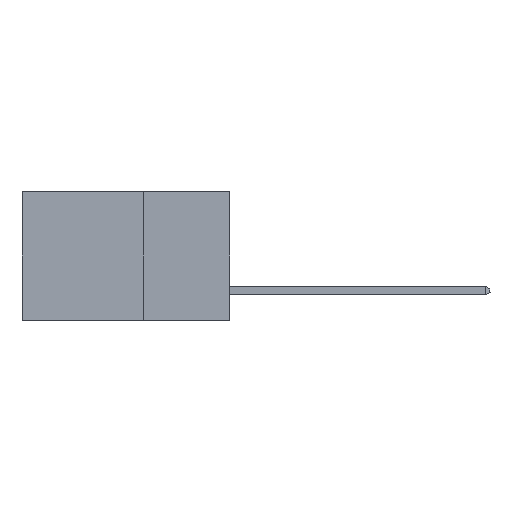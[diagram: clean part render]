
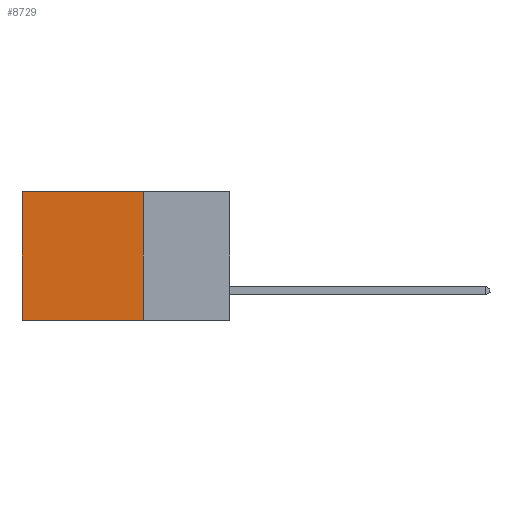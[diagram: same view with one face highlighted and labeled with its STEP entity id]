
A CAD part, left-side view. The second image highlights one B-rep face of the part: STEP entity #8729.
In plain terms, the highlighted planar face has unit normal (-1, 0, 0).
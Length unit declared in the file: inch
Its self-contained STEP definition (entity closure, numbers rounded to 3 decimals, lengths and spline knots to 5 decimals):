
#23 = EDGE_CURVE ( 'NONE', #14061, #4516, #7874, .T. ) ;
#782 = LINE ( 'NONE', #9246, #13998 ) ;
#1590 = EDGE_CURVE ( 'NONE', #4516, #4566, #14405, .T. ) ;
#2423 = LINE ( 'NONE', #7240, #13970 ) ;
#4032 = AXIS2_PLACEMENT_3D ( 'NONE', #15412, #15359, #7502 ) ;
#4516 = VERTEX_POINT ( 'NONE', #17075 ) ;
#4566 = VERTEX_POINT ( 'NONE', #12818 ) ;
#5555 = CARTESIAN_POINT ( 'NONE',  ( 0.298, 0.25, 0. ) ) ;
#7240 = CARTESIAN_POINT ( 'NONE',  ( 0.298, 0.25, -0.37 ) ) ;
#7362 = VERTEX_POINT ( 'NONE', #10658 ) ;
#7396 = VECTOR ( 'NONE', #10119, 39.37008 ) ;
#7502 = DIRECTION ( 'NONE',  ( 0., 0., -1. ) ) ;
#7874 = LINE ( 'NONE', #11354, #14892 ) ;
#8729 = ADVANCED_FACE ( 'NONE', ( #17121 ), #16239, .F. ) ;
#9246 = CARTESIAN_POINT ( 'NONE',  ( 0.298, 0.25, 0. ) ) ;
#10119 = DIRECTION ( 'NONE',  ( 0., 0., -1. ) ) ;
#10158 = DIRECTION ( 'NONE',  ( 0., 1., 0. ) ) ;
#10658 = CARTESIAN_POINT ( 'NONE',  ( 0.298, 0.25, -0.37 ) ) ;
#11211 = ORIENTED_EDGE ( 'NONE', *, *, #23, .T. ) ;
#11239 = DIRECTION ( 'NONE',  ( 0., 1., 0. ) ) ;
#11354 = CARTESIAN_POINT ( 'NONE',  ( 0.298, 0.25, 0. ) ) ;
#11490 = ORIENTED_EDGE ( 'NONE', *, *, #1590, .T. ) ;
#11975 = DIRECTION ( 'NONE',  ( 0., 0., -1. ) ) ;
#12818 = CARTESIAN_POINT ( 'NONE',  ( 0.298, 0.6, -0.37 ) ) ;
#13245 = ORIENTED_EDGE ( 'NONE', *, *, #14693, .F. ) ;
#13944 = EDGE_CURVE ( 'NONE', #14061, #7362, #782, .T. ) ;
#13970 = VECTOR ( 'NONE', #11239, 39.37008 ) ;
#13998 = VECTOR ( 'NONE', #11975, 39.37008 ) ;
#14061 = VERTEX_POINT ( 'NONE', #5555 ) ;
#14405 = LINE ( 'NONE', #15385, #7396 ) ;
#14693 = EDGE_CURVE ( 'NONE', #7362, #4566, #2423, .T. ) ;
#14892 = VECTOR ( 'NONE', #10158, 39.37008 ) ;
#15045 = ORIENTED_EDGE ( 'NONE', *, *, #13944, .F. ) ;
#15359 = DIRECTION ( 'NONE',  ( 1., 0., 0. ) ) ;
#15385 = CARTESIAN_POINT ( 'NONE',  ( 0.298, 0.6, 0. ) ) ;
#15412 = CARTESIAN_POINT ( 'NONE',  ( 0.298, 0.25, 0. ) ) ;
#15705 = EDGE_LOOP ( 'NONE', ( #11490, #13245, #15045, #11211 ) ) ;
#16239 = PLANE ( 'NONE',  #4032 ) ;
#17075 = CARTESIAN_POINT ( 'NONE',  ( 0.298, 0.6, 0. ) ) ;
#17121 = FACE_OUTER_BOUND ( 'NONE', #15705, .T. ) ;
